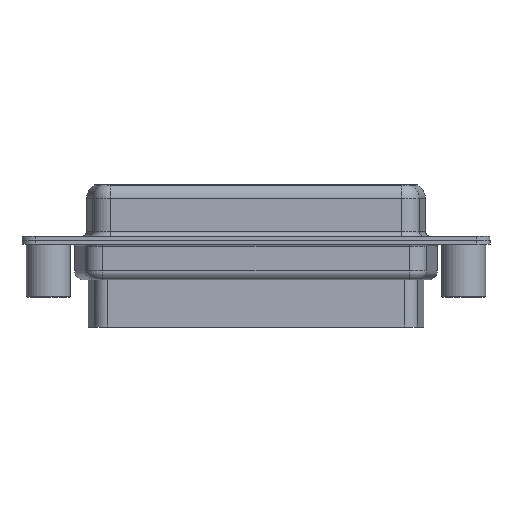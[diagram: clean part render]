
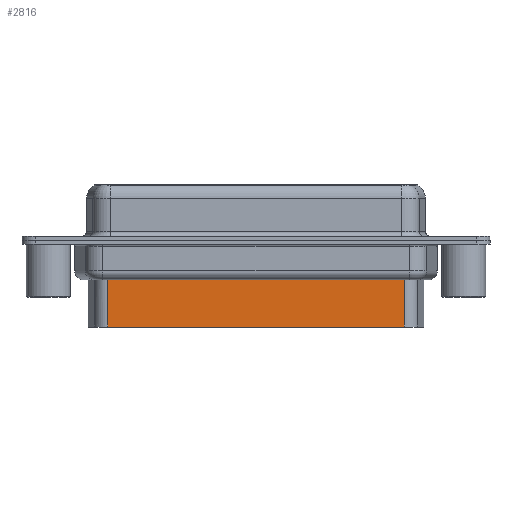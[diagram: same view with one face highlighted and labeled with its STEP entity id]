
A CAD part, front view. The second image highlights one B-rep face of the part: STEP entity #2816.
In plain terms, the highlighted planar face has unit normal (0, -1, 0).
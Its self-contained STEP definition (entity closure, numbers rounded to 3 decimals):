
#230 = CARTESIAN_POINT ( 'NONE',  ( 40.339, -3.5, -4.097 ) ) ;
#605 = CARTESIAN_POINT ( 'NONE',  ( 6.701, -3.5, -9.85 ) ) ;
#1018 = ORIENTED_EDGE ( 'NONE', *, *, #16877, .F. ) ;
#2816 = ADVANCED_FACE ( 'NONE', ( #2989 ), #25012, .T. ) ;
#2989 = FACE_OUTER_BOUND ( 'NONE', #21612, .T. ) ;
#4732 = VECTOR ( 'NONE', #16822, 1000. ) ;
#4962 = CARTESIAN_POINT ( 'NONE',  ( 6.701, -3.5, -3.1 ) ) ;
#5331 = EDGE_CURVE ( 'NONE', #20039, #17774, #16956, .T. ) ;
#7119 = CARTESIAN_POINT ( 'NONE',  ( 6.454, -3.5, -4.097 ) ) ;
#7307 = DIRECTION ( 'NONE',  ( 0., -1., 0. ) ) ;
#7966 = VECTOR ( 'NONE', #20773, 1000. ) ;
#8098 = CARTESIAN_POINT ( 'NONE',  ( 40.339, -3.5, -3.1 ) ) ;
#8716 = LINE ( 'NONE', #7119, #4732 ) ;
#9527 = ORIENTED_EDGE ( 'NONE', *, *, #5331, .T. ) ;
#10322 = DIRECTION ( 'NONE',  ( 0., 0., -1. ) ) ;
#10873 = DIRECTION ( 'NONE',  ( 1., 0., 0. ) ) ;
#11880 = VERTEX_POINT ( 'NONE', #24029 ) ;
#12284 = DIRECTION ( 'NONE',  ( -1., 0., 0. ) ) ;
#13867 = AXIS2_PLACEMENT_3D ( 'NONE', #4962, #7307, #10873 ) ;
#14038 = CARTESIAN_POINT ( 'NONE',  ( 6.701, -3.5, -9.85 ) ) ;
#16714 = CARTESIAN_POINT ( 'NONE',  ( 6.701, -3.5, -3.1 ) ) ;
#16822 = DIRECTION ( 'NONE',  ( -1., 0., 0. ) ) ;
#16877 = EDGE_CURVE ( 'NONE', #11880, #17774, #20655, .T. ) ;
#16956 = LINE ( 'NONE', #16714, #7966 ) ;
#17252 = VECTOR ( 'NONE', #10322, 1000. ) ;
#17774 = VERTEX_POINT ( 'NONE', #14038 ) ;
#17910 = ORIENTED_EDGE ( 'NONE', *, *, #20466, .T. ) ;
#18049 = LINE ( 'NONE', #8098, #17252 ) ;
#18234 = EDGE_CURVE ( 'NONE', #25462, #11880, #18049, .T. ) ;
#20039 = VERTEX_POINT ( 'NONE', #24599 ) ;
#20466 = EDGE_CURVE ( 'NONE', #25462, #20039, #8716, .T. ) ;
#20655 = LINE ( 'NONE', #605, #24213 ) ;
#20773 = DIRECTION ( 'NONE',  ( 0., 0., -1. ) ) ;
#21612 = EDGE_LOOP ( 'NONE', ( #23801, #17910, #9527, #1018 ) ) ;
#23801 = ORIENTED_EDGE ( 'NONE', *, *, #18234, .F. ) ;
#24029 = CARTESIAN_POINT ( 'NONE',  ( 40.339, -3.5, -9.85 ) ) ;
#24213 = VECTOR ( 'NONE', #12284, 1000. ) ;
#24599 = CARTESIAN_POINT ( 'NONE',  ( 6.701, -3.5, -4.097 ) ) ;
#25012 = PLANE ( 'NONE',  #13867 ) ;
#25462 = VERTEX_POINT ( 'NONE', #230 ) ;
